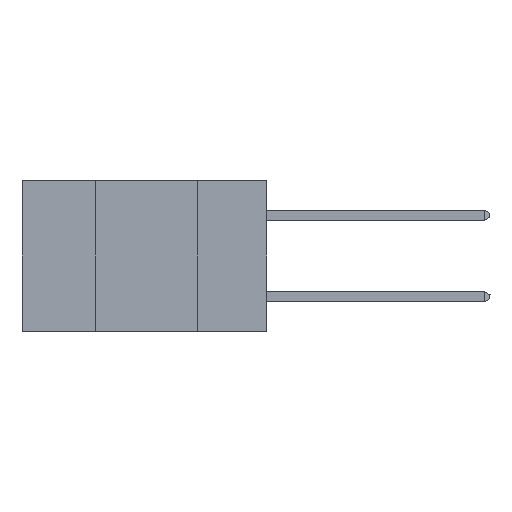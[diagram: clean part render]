
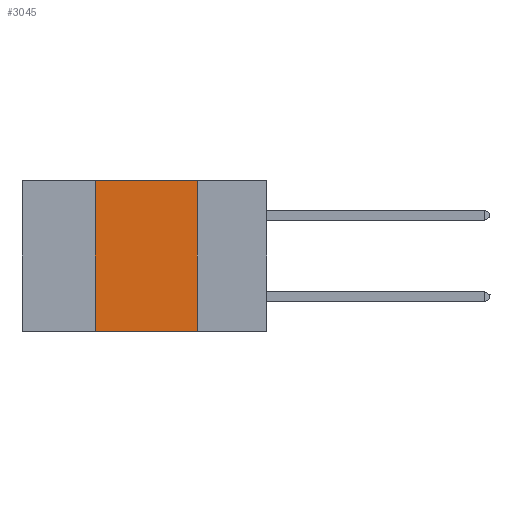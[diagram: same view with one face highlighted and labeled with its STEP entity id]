
A CAD part, left-side view. The second image highlights one B-rep face of the part: STEP entity #3045.
In plain terms, the highlighted planar face has unit normal (-1, 0, 0).
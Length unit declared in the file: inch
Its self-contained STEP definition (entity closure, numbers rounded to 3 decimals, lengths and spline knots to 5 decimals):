
#449 = VERTEX_POINT ( 'NONE', #17413 ) ;
#1104 = DIRECTION ( 'NONE',  ( 0., 0., 1. ) ) ;
#1210 = EDGE_CURVE ( 'NONE', #449, #4591, #9131, .T. ) ;
#1415 = EDGE_CURVE ( 'NONE', #2307, #4591, #18417, .T. ) ;
#1818 = DIRECTION ( 'NONE',  ( 0., 0., -1. ) ) ;
#2058 = EDGE_CURVE ( 'NONE', #449, #21207, #9087, .T. ) ;
#2307 = VERTEX_POINT ( 'NONE', #16528 ) ;
#2372 = VECTOR ( 'NONE', #10787, 39.37008 ) ;
#2402 = CARTESIAN_POINT ( 'NONE',  ( 0., 0.6, 0. ) ) ;
#2581 = FACE_OUTER_BOUND ( 'NONE', #18492, .T. ) ;
#3045 = ADVANCED_FACE ( 'NONE', ( #2581 ), #6591, .F. ) ;
#3112 = CARTESIAN_POINT ( 'NONE',  ( 0., 0.17, 0. ) ) ;
#3144 = DIRECTION ( 'NONE',  ( 1., 0., 0. ) ) ;
#4591 = VERTEX_POINT ( 'NONE', #10298 ) ;
#4914 = ORIENTED_EDGE ( 'NONE', *, *, #1415, .F. ) ;
#6311 = CARTESIAN_POINT ( 'NONE',  ( 0., 0.42, 0. ) ) ;
#6591 = PLANE ( 'NONE',  #18934 ) ;
#7816 = EDGE_CURVE ( 'NONE', #21207, #2307, #13721, .T. ) ;
#7950 = ORIENTED_EDGE ( 'NONE', *, *, #2058, .F. ) ;
#8059 = CARTESIAN_POINT ( 'NONE',  ( 0., 0.6, 0. ) ) ;
#9014 = CARTESIAN_POINT ( 'NONE',  ( 0., 0.42, 0. ) ) ;
#9087 = LINE ( 'NONE', #6311, #18381 ) ;
#9131 = LINE ( 'NONE', #14718, #10691 ) ;
#10298 = CARTESIAN_POINT ( 'NONE',  ( 0., 0.17, -0.37 ) ) ;
#10691 = VECTOR ( 'NONE', #16383, 39.37008 ) ;
#10787 = DIRECTION ( 'NONE',  ( 0., -1., 0. ) ) ;
#10934 = VECTOR ( 'NONE', #21034, 39.37008 ) ;
#13231 = ORIENTED_EDGE ( 'NONE', *, *, #7816, .F. ) ;
#13721 = LINE ( 'NONE', #2402, #2372 ) ;
#14718 = CARTESIAN_POINT ( 'NONE',  ( 0., 0.6, -0.37 ) ) ;
#16383 = DIRECTION ( 'NONE',  ( 0., -1., 0. ) ) ;
#16528 = CARTESIAN_POINT ( 'NONE',  ( 0., 0.17, 0. ) ) ;
#16603 = ORIENTED_EDGE ( 'NONE', *, *, #1210, .T. ) ;
#17413 = CARTESIAN_POINT ( 'NONE',  ( 0., 0.42, -0.37 ) ) ;
#18381 = VECTOR ( 'NONE', #1104, 39.37008 ) ;
#18417 = LINE ( 'NONE', #3112, #10934 ) ;
#18492 = EDGE_LOOP ( 'NONE', ( #4914, #13231, #7950, #16603 ) ) ;
#18934 = AXIS2_PLACEMENT_3D ( 'NONE', #8059, #3144, #1818 ) ;
#21034 = DIRECTION ( 'NONE',  ( 0., 0., -1. ) ) ;
#21207 = VERTEX_POINT ( 'NONE', #9014 ) ;
